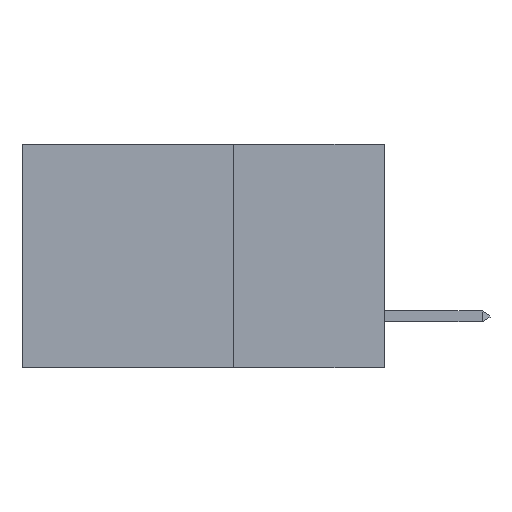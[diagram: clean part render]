
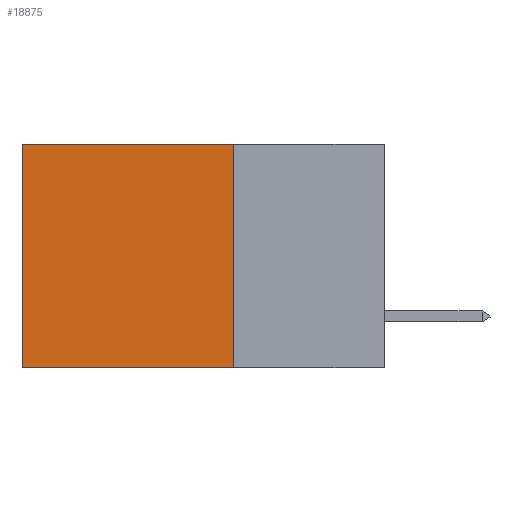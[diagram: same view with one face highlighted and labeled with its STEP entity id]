
A CAD part, left-side view. The second image highlights one B-rep face of the part: STEP entity #18875.
In plain terms, the highlighted planar face has unit normal (-1, 0, 0).
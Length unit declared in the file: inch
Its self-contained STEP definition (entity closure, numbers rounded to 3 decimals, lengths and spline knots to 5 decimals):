
#953 = DIRECTION ( 'NONE',  ( 0., 0., -1. ) ) ;
#2813 = CARTESIAN_POINT ( 'NONE',  ( 0.2875, 0.25, 0. ) ) ;
#2853 = CARTESIAN_POINT ( 'NONE',  ( 0.2875, 0.25, 0. ) ) ;
#3014 = FACE_OUTER_BOUND ( 'NONE', #15513, .T. ) ;
#3068 = ORIENTED_EDGE ( 'NONE', *, *, #16330, .T. ) ;
#4793 = ORIENTED_EDGE ( 'NONE', *, *, #16896, .F. ) ;
#4818 = DIRECTION ( 'NONE',  ( 0., 0., -1. ) ) ;
#5618 = ORIENTED_EDGE ( 'NONE', *, *, #20878, .T. ) ;
#7503 = VERTEX_POINT ( 'NONE', #18792 ) ;
#7536 = LINE ( 'NONE', #20217, #16751 ) ;
#7721 = VECTOR ( 'NONE', #953, 39.37008 ) ;
#8055 = DIRECTION ( 'NONE',  ( 0., 1., 0. ) ) ;
#10251 = DIRECTION ( 'NONE',  ( 0., 1., 0. ) ) ;
#10632 = PLANE ( 'NONE',  #12933 ) ;
#10666 = CARTESIAN_POINT ( 'NONE',  ( 0.2875, 0.6, 0. ) ) ;
#11360 = CARTESIAN_POINT ( 'NONE',  ( 0.2875, 0.6, 0. ) ) ;
#11917 = CARTESIAN_POINT ( 'NONE',  ( 0.2875, 0.25, -0.37 ) ) ;
#12017 = LINE ( 'NONE', #11360, #21991 ) ;
#12339 = VERTEX_POINT ( 'NONE', #10666 ) ;
#12933 = AXIS2_PLACEMENT_3D ( 'NONE', #2853, #16563, #4818 ) ;
#13350 = DIRECTION ( 'NONE',  ( 0., 0., -1. ) ) ;
#13372 = EDGE_CURVE ( 'NONE', #15174, #7503, #19960, .T. ) ;
#14638 = VECTOR ( 'NONE', #8055, 39.37008 ) ;
#14872 = VERTEX_POINT ( 'NONE', #2813 ) ;
#15174 = VERTEX_POINT ( 'NONE', #11917 ) ;
#15513 = EDGE_LOOP ( 'NONE', ( #3068, #19828, #4793, #5618 ) ) ;
#16330 = EDGE_CURVE ( 'NONE', #12339, #7503, #12017, .T. ) ;
#16563 = DIRECTION ( 'NONE',  ( 1., 0., 0. ) ) ;
#16570 = CARTESIAN_POINT ( 'NONE',  ( 0.2875, 0.25, 0. ) ) ;
#16751 = VECTOR ( 'NONE', #10251, 39.37008 ) ;
#16896 = EDGE_CURVE ( 'NONE', #14872, #15174, #24121, .T. ) ;
#18792 = CARTESIAN_POINT ( 'NONE',  ( 0.2875, 0.6, -0.37 ) ) ;
#18875 = ADVANCED_FACE ( 'NONE', ( #3014 ), #10632, .F. ) ;
#19828 = ORIENTED_EDGE ( 'NONE', *, *, #13372, .F. ) ;
#19905 = CARTESIAN_POINT ( 'NONE',  ( 0.2875, 0.25, -0.37 ) ) ;
#19960 = LINE ( 'NONE', #19905, #14638 ) ;
#20217 = CARTESIAN_POINT ( 'NONE',  ( 0.2875, 0.25, 0. ) ) ;
#20878 = EDGE_CURVE ( 'NONE', #14872, #12339, #7536, .T. ) ;
#21991 = VECTOR ( 'NONE', #13350, 39.37008 ) ;
#24121 = LINE ( 'NONE', #16570, #7721 ) ;
